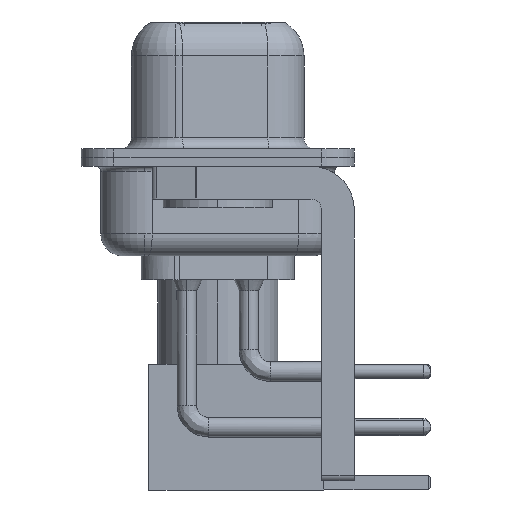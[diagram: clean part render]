
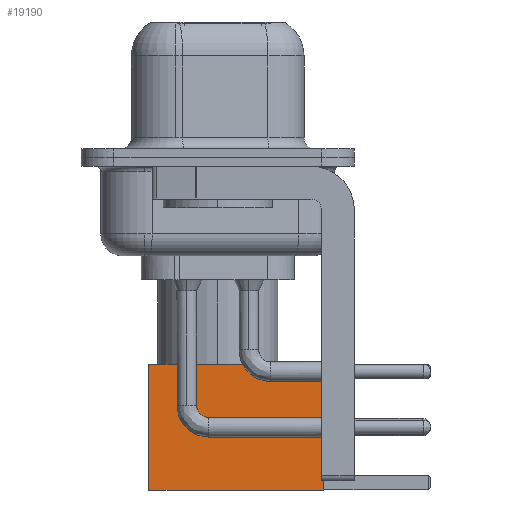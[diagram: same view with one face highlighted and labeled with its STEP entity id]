
A CAD part, left-side view. The second image highlights one B-rep face of the part: STEP entity #19190.
In plain terms, the highlighted face is planar.
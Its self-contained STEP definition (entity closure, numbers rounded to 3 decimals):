
#150 = CARTESIAN_POINT ( 'NONE',  ( 0., 2.875, 8. ) ) ;
#698 = ORIENTED_EDGE ( 'NONE', *, *, #9626, .F. ) ;
#705 = EDGE_CURVE ( 'NONE', #2689, #16239, #13414, .T. ) ;
#946 = CARTESIAN_POINT ( 'NONE',  ( 0., 2.875, 0. ) ) ;
#2309 = VECTOR ( 'NONE', #16107, 1000. ) ;
#2689 = VERTEX_POINT ( 'NONE', #13687 ) ;
#3002 = LINE ( 'NONE', #150, #5865 ) ;
#3030 = CARTESIAN_POINT ( 'NONE',  ( -2.875, 2.875, 0. ) ) ;
#3269 = CARTESIAN_POINT ( 'NONE',  ( -2.875, 2.875, 0. ) ) ;
#3327 = LINE ( 'NONE', #3030, #8899 ) ;
#4759 = CARTESIAN_POINT ( 'NONE',  ( 2.875, 2.875, 8. ) ) ;
#5155 = LINE ( 'NONE', #17748, #2309 ) ;
#5865 = VECTOR ( 'NONE', #6381, 1000. ) ;
#6381 = DIRECTION ( 'NONE',  ( -1., 0., 0. ) ) ;
#6486 = ORIENTED_EDGE ( 'NONE', *, *, #705, .T. ) ;
#6680 = FACE_OUTER_BOUND ( 'NONE', #19748, .T. ) ;
#6707 = VERTEX_POINT ( 'NONE', #4759 ) ;
#7298 = ORIENTED_EDGE ( 'NONE', *, *, #14621, .F. ) ;
#8208 = CARTESIAN_POINT ( 'NONE',  ( 2.875, 2.875, 0. ) ) ;
#8788 = DIRECTION ( 'NONE',  ( -1., 0., 0. ) ) ;
#8899 = VECTOR ( 'NONE', #12742, 1000. ) ;
#9626 = EDGE_CURVE ( 'NONE', #6707, #18631, #3002, .T. ) ;
#9636 = DIRECTION ( 'NONE',  ( 0., 0., 1. ) ) ;
#10025 = AXIS2_PLACEMENT_3D ( 'NONE', #8208, #15700, #9636 ) ;
#11095 = EDGE_CURVE ( 'NONE', #6707, #2689, #5155, .T. ) ;
#12553 = ORIENTED_EDGE ( 'NONE', *, *, #11095, .T. ) ;
#12624 = PLANE ( 'NONE',  #10025 ) ;
#12740 = VECTOR ( 'NONE', #8788, 1000. ) ;
#12742 = DIRECTION ( 'NONE',  ( 0., 0., -1. ) ) ;
#13414 = LINE ( 'NONE', #946, #12740 ) ;
#13687 = CARTESIAN_POINT ( 'NONE',  ( 2.875, 2.875, 0. ) ) ;
#14621 = EDGE_CURVE ( 'NONE', #18631, #16239, #3327, .T. ) ;
#15700 = DIRECTION ( 'NONE',  ( 0., 1., 0. ) ) ;
#16107 = DIRECTION ( 'NONE',  ( 0., 0., -1. ) ) ;
#16239 = VERTEX_POINT ( 'NONE', #3269 ) ;
#17748 = CARTESIAN_POINT ( 'NONE',  ( 2.875, 2.875, 0. ) ) ;
#18502 = CARTESIAN_POINT ( 'NONE',  ( -2.875, 2.875, 8. ) ) ;
#18631 = VERTEX_POINT ( 'NONE', #18502 ) ;
#19190 = ADVANCED_FACE ( 'NONE', ( #6680 ), #12624, .T. ) ;
#19748 = EDGE_LOOP ( 'NONE', ( #12553, #6486, #7298, #698 ) ) ;
